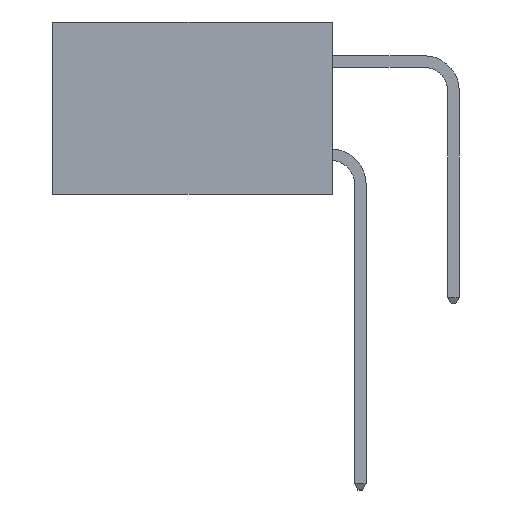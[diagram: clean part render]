
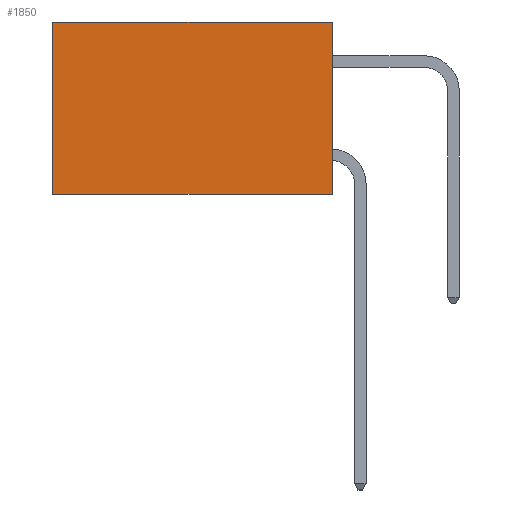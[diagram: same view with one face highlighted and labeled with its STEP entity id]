
A CAD part, left-side view. The second image highlights one B-rep face of the part: STEP entity #1850.
In plain terms, the highlighted planar face has unit normal (-1, 0, 0).
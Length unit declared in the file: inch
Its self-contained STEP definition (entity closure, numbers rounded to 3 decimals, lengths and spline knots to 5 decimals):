
#518 = DIRECTION ( 'NONE',  ( 1., 0., 0. ) ) ;
#563 = EDGE_CURVE ( 'NONE', #12199, #10603, #6976, .T. ) ;
#802 = ORIENTED_EDGE ( 'NONE', *, *, #563, .F. ) ;
#876 = ORIENTED_EDGE ( 'NONE', *, *, #4472, .T. ) ;
#1139 = AXIS2_PLACEMENT_3D ( 'NONE', #2490, #518, #7626 ) ;
#1201 = CARTESIAN_POINT ( 'NONE',  ( 0.2615, 0.6, -0.37 ) ) ;
#1627 = VECTOR ( 'NONE', #7805, 39.37008 ) ;
#1753 = VECTOR ( 'NONE', #4719, 39.37008 ) ;
#1850 = ADVANCED_FACE ( 'NONE', ( #3514 ), #6616, .F. ) ;
#1982 = CARTESIAN_POINT ( 'NONE',  ( 0.2615, 0., 0. ) ) ;
#2056 = CARTESIAN_POINT ( 'NONE',  ( 0.2615, 0., -0.37 ) ) ;
#2268 = CARTESIAN_POINT ( 'NONE',  ( 0.2615, 0., -0.37 ) ) ;
#2490 = CARTESIAN_POINT ( 'NONE',  ( 0.2615, 0., -0.37 ) ) ;
#2536 = CARTESIAN_POINT ( 'NONE',  ( 0.2615, 0., -0.37 ) ) ;
#3514 = FACE_OUTER_BOUND ( 'NONE', #8388, .T. ) ;
#3689 = CARTESIAN_POINT ( 'NONE',  ( 0.2615, 0.6, -0.37 ) ) ;
#3927 = LINE ( 'NONE', #12849, #9253 ) ;
#3983 = ORIENTED_EDGE ( 'NONE', *, *, #12518, .F. ) ;
#4472 = EDGE_CURVE ( 'NONE', #5786, #7656, #3927, .T. ) ;
#4692 = CARTESIAN_POINT ( 'NONE',  ( 0.2615, 0.6, 0. ) ) ;
#4719 = DIRECTION ( 'NONE',  ( 0., 0., -1. ) ) ;
#5786 = VERTEX_POINT ( 'NONE', #1982 ) ;
#6141 = DIRECTION ( 'NONE',  ( 0., 0., -1. ) ) ;
#6171 = ORIENTED_EDGE ( 'NONE', *, *, #8336, .T. ) ;
#6616 = PLANE ( 'NONE',  #1139 ) ;
#6808 = DIRECTION ( 'NONE',  ( 0., 1., 0. ) ) ;
#6976 = LINE ( 'NONE', #2268, #1627 ) ;
#7626 = DIRECTION ( 'NONE',  ( 0., 0., -1. ) ) ;
#7656 = VERTEX_POINT ( 'NONE', #4692 ) ;
#7805 = DIRECTION ( 'NONE',  ( 0., 1., 0. ) ) ;
#8336 = EDGE_CURVE ( 'NONE', #7656, #10603, #9796, .T. ) ;
#8388 = EDGE_LOOP ( 'NONE', ( #6171, #802, #3983, #876 ) ) ;
#8885 = VECTOR ( 'NONE', #6141, 39.37008 ) ;
#9253 = VECTOR ( 'NONE', #6808, 39.37008 ) ;
#9796 = LINE ( 'NONE', #3689, #1753 ) ;
#10603 = VERTEX_POINT ( 'NONE', #1201 ) ;
#11565 = LINE ( 'NONE', #2056, #8885 ) ;
#12199 = VERTEX_POINT ( 'NONE', #2536 ) ;
#12518 = EDGE_CURVE ( 'NONE', #5786, #12199, #11565, .T. ) ;
#12849 = CARTESIAN_POINT ( 'NONE',  ( 0.2615, 0., 0. ) ) ;
